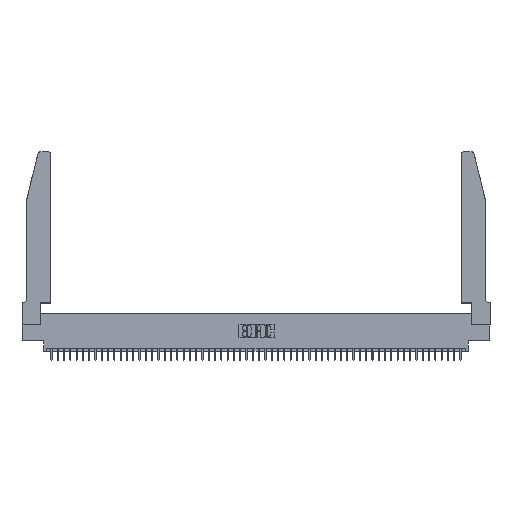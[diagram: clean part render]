
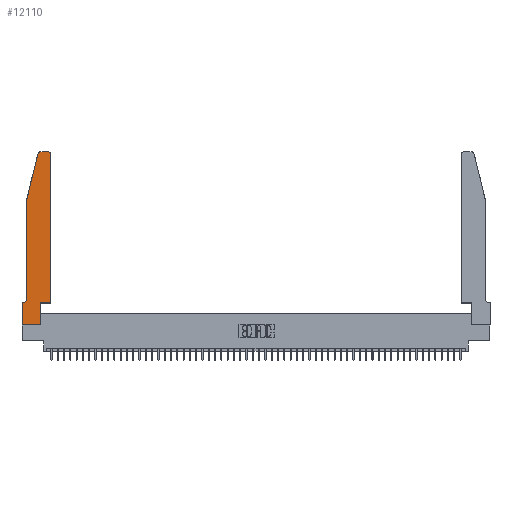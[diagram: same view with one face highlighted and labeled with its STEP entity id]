
A CAD part, top view. The second image highlights one B-rep face of the part: STEP entity #12110.
In plain terms, the highlighted planar face has unit normal (0, 0, 1).
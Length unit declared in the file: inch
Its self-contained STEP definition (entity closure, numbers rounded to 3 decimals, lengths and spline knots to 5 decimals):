
#173 = EDGE_CURVE ( 'NONE', #47985, #36960, #16804, .T. ) ;
#851 = CIRCLE ( 'NONE', #32897, 0.07 ) ;
#904 = LINE ( 'NONE', #30135, #18712 ) ;
#2343 = VECTOR ( 'NONE', #23121, 39.37008 ) ;
#3309 = VERTEX_POINT ( 'NONE', #14187 ) ;
#4039 = CARTESIAN_POINT ( 'NONE',  ( 0.284, 2.72, 0.37 ) ) ;
#6394 = PLANE ( 'NONE',  #15494 ) ;
#7476 = EDGE_CURVE ( 'NONE', #41286, #3309, #10155, .T. ) ;
#7575 = VERTEX_POINT ( 'NONE', #53241 ) ;
#8353 = DIRECTION ( 'NONE',  ( 1., 0., 0. ) ) ;
#9382 = ORIENTED_EDGE ( 'NONE', *, *, #30836, .T. ) ;
#9563 = ORIENTED_EDGE ( 'NONE', *, *, #38314, .T. ) ;
#10155 = LINE ( 'NONE', #44039, #2343 ) ;
#11221 = VERTEX_POINT ( 'NONE', #38597 ) ;
#11938 = LINE ( 'NONE', #36631, #31644 ) ;
#12110 = ADVANCED_FACE ( 'NONE', ( #31299 ), #6394, .T. ) ;
#14187 = CARTESIAN_POINT ( 'NONE',  ( 0.0755, 2., 0.37 ) ) ;
#14279 = CARTESIAN_POINT ( 'NONE',  ( 0.0055, 0.35, 0.37 ) ) ;
#14856 = DIRECTION ( 'NONE',  ( -1., 0., 0. ) ) ;
#15454 = CARTESIAN_POINT ( 'NONE',  ( 0.2865, 0.35, 0.37 ) ) ;
#15494 = AXIS2_PLACEMENT_3D ( 'NONE', #52206, #30742, #35372 ) ;
#16420 = EDGE_CURVE ( 'NONE', #51327, #32329, #11938, .T. ) ;
#16487 = CIRCLE ( 'NONE', #43371, 0.03 ) ;
#16559 = ORIENTED_EDGE ( 'NONE', *, *, #42268, .T. ) ;
#16804 = LINE ( 'NONE', #29011, #27637 ) ;
#17026 = CARTESIAN_POINT ( 'NONE',  ( 0.2865, 0., 0.37 ) ) ;
#17187 = ORIENTED_EDGE ( 'NONE', *, *, #48385, .T. ) ;
#17586 = EDGE_CURVE ( 'NONE', #7575, #47985, #34724, .T. ) ;
#17948 = DIRECTION ( 'NONE',  ( 0., -1., 0. ) ) ;
#18712 = VECTOR ( 'NONE', #17948, 39.37008 ) ;
#18966 = DIRECTION ( 'NONE',  ( 1., 0., 0. ) ) ;
#18987 = VECTOR ( 'NONE', #48127, 39.37008 ) ;
#20056 = VERTEX_POINT ( 'NONE', #37110 ) ;
#20122 = CIRCLE ( 'NONE', #27051, 0.03 ) ;
#20421 = ORIENTED_EDGE ( 'NONE', *, *, #22165, .T. ) ;
#20995 = ORIENTED_EDGE ( 'NONE', *, *, #173, .T. ) ;
#21146 = CARTESIAN_POINT ( 'NONE',  ( 0.4205, 2.72, 0.37 ) ) ;
#22165 = EDGE_CURVE ( 'NONE', #36960, #51327, #23391, .T. ) ;
#22217 = DIRECTION ( 'NONE',  ( 1., 0., 0. ) ) ;
#22688 = VERTEX_POINT ( 'NONE', #39736 ) ;
#22719 = EDGE_LOOP ( 'NONE', ( #9382, #16559, #25131, #17187, #43351, #52935, #34744, #20995, #20421, #23273, #36490, #9563 ) ) ;
#22989 = EDGE_CURVE ( 'NONE', #32329, #20056, #38055, .T. ) ;
#23049 = CARTESIAN_POINT ( 'NONE',  ( 0., 0., 0.37 ) ) ;
#23121 = DIRECTION ( 'NONE',  ( -0.239, -0.971, 0. ) ) ;
#23273 = ORIENTED_EDGE ( 'NONE', *, *, #16420, .T. ) ;
#23391 = LINE ( 'NONE', #40009, #18987 ) ;
#25131 = ORIENTED_EDGE ( 'NONE', *, *, #7476, .T. ) ;
#25626 = VECTOR ( 'NONE', #43422, 39.37008 ) ;
#27051 = AXIS2_PLACEMENT_3D ( 'NONE', #4039, #45758, #8353 ) ;
#27637 = VECTOR ( 'NONE', #29269, 39.37008 ) ;
#27658 = DIRECTION ( 'NONE',  ( -1., 0., 0. ) ) ;
#27712 = VERTEX_POINT ( 'NONE', #14279 ) ;
#28957 = CARTESIAN_POINT ( 'NONE',  ( 0., 0., 0.37 ) ) ;
#29011 = CARTESIAN_POINT ( 'NONE',  ( 0., 0., 0.37 ) ) ;
#29269 = DIRECTION ( 'NONE',  ( 1., 0., 0. ) ) ;
#29823 = DIRECTION ( 'NONE',  ( 0., 0., 1. ) ) ;
#30135 = CARTESIAN_POINT ( 'NONE',  ( 0.0755, 2., 0.37 ) ) ;
#30742 = DIRECTION ( 'NONE',  ( 0., 0., 1. ) ) ;
#30836 = EDGE_CURVE ( 'NONE', #52127, #22688, #50272, .T. ) ;
#31299 = FACE_OUTER_BOUND ( 'NONE', #22719, .T. ) ;
#31644 = VECTOR ( 'NONE', #18966, 39.37008 ) ;
#32214 = LINE ( 'NONE', #52043, #39234 ) ;
#32329 = VERTEX_POINT ( 'NONE', #39957 ) ;
#32897 = AXIS2_PLACEMENT_3D ( 'NONE', #39403, #34735, #27658 ) ;
#34724 = LINE ( 'NONE', #23049, #25626 ) ;
#34735 = DIRECTION ( 'NONE',  ( 0., 0., -1. ) ) ;
#34744 = ORIENTED_EDGE ( 'NONE', *, *, #17586, .T. ) ;
#35372 = DIRECTION ( 'NONE',  ( 1., 0., 0. ) ) ;
#36490 = ORIENTED_EDGE ( 'NONE', *, *, #22989, .T. ) ;
#36631 = CARTESIAN_POINT ( 'NONE',  ( 0.4505, 0.35, 0.37 ) ) ;
#36960 = VERTEX_POINT ( 'NONE', #17026 ) ;
#36988 = CARTESIAN_POINT ( 'NONE',  ( 0.4205, 2.75, 0.37 ) ) ;
#37110 = CARTESIAN_POINT ( 'NONE',  ( 0.4505, 2.72, 0.37 ) ) ;
#38055 = LINE ( 'NONE', #50530, #40625 ) ;
#38314 = EDGE_CURVE ( 'NONE', #20056, #52127, #16487, .T. ) ;
#38597 = CARTESIAN_POINT ( 'NONE',  ( 0.0755, 0.42, 0.37 ) ) ;
#39234 = VECTOR ( 'NONE', #14856, 39.37008 ) ;
#39403 = CARTESIAN_POINT ( 'NONE',  ( 0.0055, 0.42, 0.37 ) ) ;
#39736 = CARTESIAN_POINT ( 'NONE',  ( 0.284, 2.75, 0.37 ) ) ;
#39957 = CARTESIAN_POINT ( 'NONE',  ( 0.4505, 0.35, 0.37 ) ) ;
#40009 = CARTESIAN_POINT ( 'NONE',  ( 0.2865, 0.35, 0.37 ) ) ;
#40625 = VECTOR ( 'NONE', #47250, 39.37008 ) ;
#41286 = VERTEX_POINT ( 'NONE', #50896 ) ;
#42156 = EDGE_CURVE ( 'NONE', #27712, #7575, #32214, .T. ) ;
#42268 = EDGE_CURVE ( 'NONE', #22688, #41286, #20122, .T. ) ;
#43351 = ORIENTED_EDGE ( 'NONE', *, *, #52522, .T. ) ;
#43371 = AXIS2_PLACEMENT_3D ( 'NONE', #21146, #29823, #22217 ) ;
#43422 = DIRECTION ( 'NONE',  ( 0., -1., 0. ) ) ;
#44039 = CARTESIAN_POINT ( 'NONE',  ( 0.0755, 2., 0.37 ) ) ;
#45758 = DIRECTION ( 'NONE',  ( 0., 0., 1. ) ) ;
#46704 = CARTESIAN_POINT ( 'NONE',  ( 0.2605, 2.75, 0.37 ) ) ;
#47250 = DIRECTION ( 'NONE',  ( 0., 1., 0. ) ) ;
#47985 = VERTEX_POINT ( 'NONE', #28957 ) ;
#48127 = DIRECTION ( 'NONE',  ( 0., 1., 0. ) ) ;
#48385 = EDGE_CURVE ( 'NONE', #3309, #11221, #904, .T. ) ;
#50272 = LINE ( 'NONE', #46704, #51171 ) ;
#50530 = CARTESIAN_POINT ( 'NONE',  ( 0.4505, 0.35, 0.37 ) ) ;
#50543 = DIRECTION ( 'NONE',  ( -1., 0., 0. ) ) ;
#50896 = CARTESIAN_POINT ( 'NONE',  ( 0.25487, 2.72718, 0.37 ) ) ;
#51171 = VECTOR ( 'NONE', #50543, 39.37008 ) ;
#51327 = VERTEX_POINT ( 'NONE', #15454 ) ;
#52043 = CARTESIAN_POINT ( 'NONE',  ( 0.0755, 0.35, 0.37 ) ) ;
#52127 = VERTEX_POINT ( 'NONE', #36988 ) ;
#52206 = CARTESIAN_POINT ( 'NONE',  ( 0., 0.35, 0.37 ) ) ;
#52522 = EDGE_CURVE ( 'NONE', #11221, #27712, #851, .T. ) ;
#52935 = ORIENTED_EDGE ( 'NONE', *, *, #42156, .T. ) ;
#53241 = CARTESIAN_POINT ( 'NONE',  ( 0., 0.35, 0.37 ) ) ;
